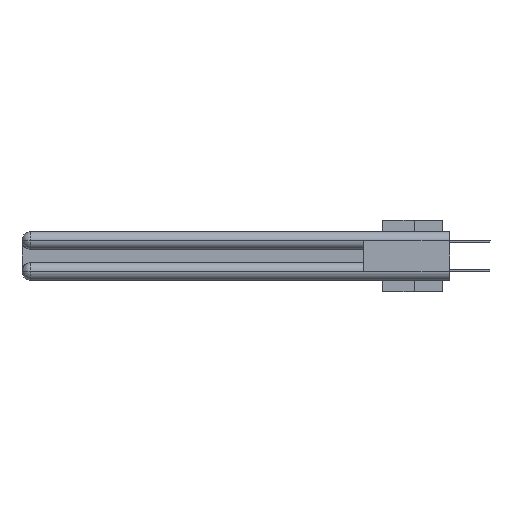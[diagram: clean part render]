
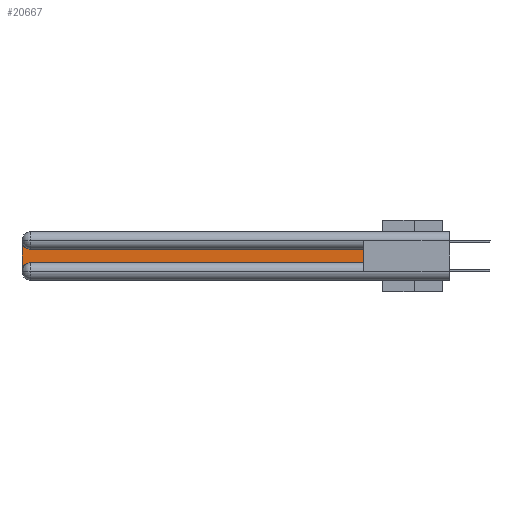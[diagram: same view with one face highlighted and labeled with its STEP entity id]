
A CAD part, left-side view. The second image highlights one B-rep face of the part: STEP entity #20667.
In plain terms, the highlighted planar face has unit normal (-1, 0, 0).
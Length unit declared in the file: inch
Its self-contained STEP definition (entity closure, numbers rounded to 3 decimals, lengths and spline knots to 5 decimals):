
#1446 = CARTESIAN_POINT ( 'NONE',  ( 0.075, 0.6, -0.2175 ) ) ;
#1496 = EDGE_CURVE ( 'NONE', #12998, #16904, #3163, .T. ) ;
#1714 = ORIENTED_EDGE ( 'NONE', *, *, #28181, .T. ) ;
#1997 = ORIENTED_EDGE ( 'NONE', *, *, #5379, .T. ) ;
#2678 = LINE ( 'NONE', #19319, #27269 ) ;
#3163 = LINE ( 'NONE', #1446, #23448 ) ;
#3448 = LINE ( 'NONE', #24934, #18605 ) ;
#3625 = CARTESIAN_POINT ( 'NONE',  ( 0.075, 3., -0.2175 ) ) ;
#4189 = FACE_OUTER_BOUND ( 'NONE', #11978, .T. ) ;
#4228 = ORIENTED_EDGE ( 'NONE', *, *, #23108, .T. ) ;
#4658 = DIRECTION ( 'NONE',  ( 0., 0., -1. ) ) ;
#4699 = DIRECTION ( 'NONE',  ( 0., -1., 0. ) ) ;
#4944 = AXIS2_PLACEMENT_3D ( 'NONE', #14117, #23958, #9758 ) ;
#5247 = CARTESIAN_POINT ( 'NONE',  ( 0.075, 2.94, -0.2175 ) ) ;
#5379 = EDGE_CURVE ( 'NONE', #16941, #20225, #15572, .T. ) ;
#6019 = ORIENTED_EDGE ( 'NONE', *, *, #8826, .T. ) ;
#8292 = DIRECTION ( 'NONE',  ( 0., 0., -1. ) ) ;
#8826 = EDGE_CURVE ( 'NONE', #20225, #29814, #10168, .T. ) ;
#9758 = DIRECTION ( 'NONE',  ( 0., 0., -1. ) ) ;
#10168 = CIRCLE ( 'NONE', #27648, 0.06 ) ;
#10893 = CIRCLE ( 'NONE', #4944, 0.06 ) ;
#11978 = EDGE_LOOP ( 'NONE', ( #4228, #21297, #1997, #6019, #1714, #27786 ) ) ;
#12364 = CARTESIAN_POINT ( 'NONE',  ( 0.075, 0.6, -0.2175 ) ) ;
#12439 = DIRECTION ( 'NONE',  ( 0., 1., 0. ) ) ;
#12998 = VERTEX_POINT ( 'NONE', #12364 ) ;
#13958 = CARTESIAN_POINT ( 'NONE',  ( 0.075, 3., -0.1225 ) ) ;
#14117 = CARTESIAN_POINT ( 'NONE',  ( 0.075, 2.94, -0.0625 ) ) ;
#14714 = EDGE_CURVE ( 'NONE', #17951, #16941, #10893, .T. ) ;
#15572 = LINE ( 'NONE', #3625, #30630 ) ;
#16295 = PLANE ( 'NONE',  #21560 ) ;
#16904 = VERTEX_POINT ( 'NONE', #21238 ) ;
#16941 = VERTEX_POINT ( 'NONE', #16994 ) ;
#16994 = CARTESIAN_POINT ( 'NONE',  ( 0.075, 3., -0.0625 ) ) ;
#17616 = DIRECTION ( 'NONE',  ( 0., 0., 1. ) ) ;
#17951 = VERTEX_POINT ( 'NONE', #29618 ) ;
#18605 = VECTOR ( 'NONE', #12439, 39.37008 ) ;
#19319 = CARTESIAN_POINT ( 'NONE',  ( 0.075, 0.6, -0.2175 ) ) ;
#19598 = CARTESIAN_POINT ( 'NONE',  ( 0.075, 2.94, -0.2775 ) ) ;
#20225 = VERTEX_POINT ( 'NONE', #26659 ) ;
#20667 = ADVANCED_FACE ( 'NONE', ( #4189 ), #16295, .F. ) ;
#21238 = CARTESIAN_POINT ( 'NONE',  ( 0.075, 0.6, -0.1225 ) ) ;
#21297 = ORIENTED_EDGE ( 'NONE', *, *, #14714, .T. ) ;
#21473 = DIRECTION ( 'NONE',  ( 0., 0., -1. ) ) ;
#21560 = AXIS2_PLACEMENT_3D ( 'NONE', #13958, #23502, #4658 ) ;
#23108 = EDGE_CURVE ( 'NONE', #16904, #17951, #3448, .T. ) ;
#23448 = VECTOR ( 'NONE', #17616, 39.37008 ) ;
#23502 = DIRECTION ( 'NONE',  ( 1., 0., 0. ) ) ;
#23958 = DIRECTION ( 'NONE',  ( 1., 0., 0. ) ) ;
#24934 = CARTESIAN_POINT ( 'NONE',  ( 0.075, 0.6, -0.1225 ) ) ;
#26177 = DIRECTION ( 'NONE',  ( 1., 0., 0. ) ) ;
#26659 = CARTESIAN_POINT ( 'NONE',  ( 0.075, 3., -0.2775 ) ) ;
#27269 = VECTOR ( 'NONE', #4699, 39.37008 ) ;
#27648 = AXIS2_PLACEMENT_3D ( 'NONE', #19598, #26177, #21473 ) ;
#27786 = ORIENTED_EDGE ( 'NONE', *, *, #1496, .T. ) ;
#28181 = EDGE_CURVE ( 'NONE', #29814, #12998, #2678, .T. ) ;
#29618 = CARTESIAN_POINT ( 'NONE',  ( 0.075, 2.94, -0.1225 ) ) ;
#29814 = VERTEX_POINT ( 'NONE', #5247 ) ;
#30630 = VECTOR ( 'NONE', #8292, 39.37008 ) ;
